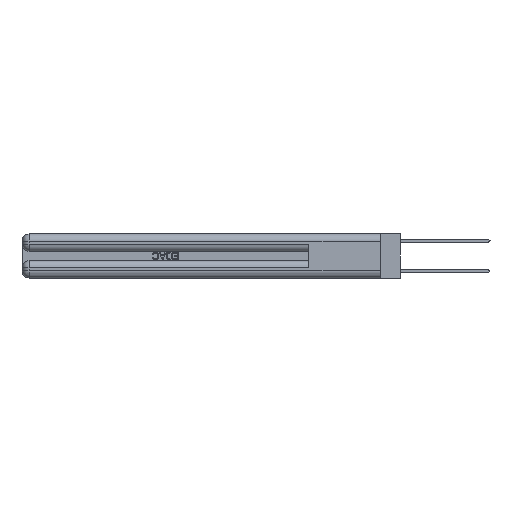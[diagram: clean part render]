
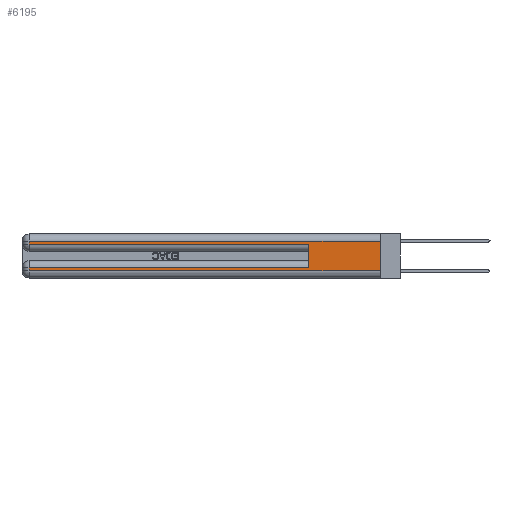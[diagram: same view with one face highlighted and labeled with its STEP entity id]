
A CAD part, left-side view. The second image highlights one B-rep face of the part: STEP entity #6195.
In plain terms, the highlighted planar face has unit normal (-1, 0, 0).
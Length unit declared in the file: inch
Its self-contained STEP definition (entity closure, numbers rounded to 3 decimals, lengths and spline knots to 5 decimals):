
#131 = VECTOR ( 'NONE', #19926, 39.37008 ) ;
#1336 = VECTOR ( 'NONE', #4763, 39.37008 ) ;
#2114 = FACE_OUTER_BOUND ( 'NONE', #22608, .T. ) ;
#2852 = ORIENTED_EDGE ( 'NONE', *, *, #32430, .T. ) ;
#2942 = CARTESIAN_POINT ( 'NONE',  ( 0., 0.6, 0.145 ) ) ;
#3414 = EDGE_CURVE ( 'NONE', #29558, #13386, #12437, .T. ) ;
#4321 = ORIENTED_EDGE ( 'NONE', *, *, #25272, .T. ) ;
#4763 = DIRECTION ( 'NONE',  ( 0., -1., 0. ) ) ;
#5176 = CARTESIAN_POINT ( 'NONE',  ( 0., 0.6, 0.085 ) ) ;
#6195 = ADVANCED_FACE ( 'NONE', ( #2114 ), #9918, .F. ) ;
#6323 = EDGE_CURVE ( 'NONE', #16266, #29972, #7254, .T. ) ;
#7254 = LINE ( 'NONE', #17371, #1336 ) ;
#7320 = ORIENTED_EDGE ( 'NONE', *, *, #3414, .T. ) ;
#8035 = ORIENTED_EDGE ( 'NONE', *, *, #6323, .T. ) ;
#8230 = DIRECTION ( 'NONE',  ( 0., 0., 1. ) ) ;
#8285 = CARTESIAN_POINT ( 'NONE',  ( 0., 2.94, 0.37 ) ) ;
#8598 = DIRECTION ( 'NONE',  ( 0., -1., 0. ) ) ;
#8967 = VERTEX_POINT ( 'NONE', #19197 ) ;
#9192 = EDGE_CURVE ( 'NONE', #29558, #8967, #27785, .T. ) ;
#9569 = VECTOR ( 'NONE', #25282, 39.37008 ) ;
#9840 = LINE ( 'NONE', #12321, #131 ) ;
#9918 = PLANE ( 'NONE',  #19857 ) ;
#9964 = CARTESIAN_POINT ( 'NONE',  ( 0., 0., 0.085 ) ) ;
#10027 = CARTESIAN_POINT ( 'NONE',  ( 0., 2.94, 0.085 ) ) ;
#10107 = VECTOR ( 'NONE', #22360, 39.37008 ) ;
#10209 = VERTEX_POINT ( 'NONE', #16473 ) ;
#10332 = DIRECTION ( 'NONE',  ( 0., 0., -1. ) ) ;
#10405 = LINE ( 'NONE', #15063, #14981 ) ;
#10663 = VECTOR ( 'NONE', #25517, 39.37008 ) ;
#10848 = CARTESIAN_POINT ( 'NONE',  ( 0., 2.94, 0.285 ) ) ;
#12321 = CARTESIAN_POINT ( 'NONE',  ( 0., 2.94, 0.37 ) ) ;
#12437 = LINE ( 'NONE', #9964, #10107 ) ;
#12543 = LINE ( 'NONE', #30387, #9569 ) ;
#13386 = VERTEX_POINT ( 'NONE', #10027 ) ;
#14399 = ORIENTED_EDGE ( 'NONE', *, *, #9192, .F. ) ;
#14981 = VECTOR ( 'NONE', #10332, 39.37008 ) ;
#15063 = CARTESIAN_POINT ( 'NONE',  ( 0., 0., 0.37 ) ) ;
#16266 = VERTEX_POINT ( 'NONE', #28032 ) ;
#16473 = CARTESIAN_POINT ( 'NONE',  ( 0., 2.94, 0.31 ) ) ;
#17123 = VERTEX_POINT ( 'NONE', #18314 ) ;
#17371 = CARTESIAN_POINT ( 'NONE',  ( 0., 0., 0.06 ) ) ;
#17834 = VECTOR ( 'NONE', #8598, 39.37008 ) ;
#18314 = CARTESIAN_POINT ( 'NONE',  ( 0., 0., 0.31 ) ) ;
#19032 = LINE ( 'NONE', #28629, #17834 ) ;
#19197 = CARTESIAN_POINT ( 'NONE',  ( 0., 0.6, 0.285 ) ) ;
#19857 = AXIS2_PLACEMENT_3D ( 'NONE', #24818, #22485, #25458 ) ;
#19926 = DIRECTION ( 'NONE',  ( 0., 0., -1. ) ) ;
#21471 = VECTOR ( 'NONE', #8230, 39.37008 ) ;
#21718 = CARTESIAN_POINT ( 'NONE',  ( 0., 0., 0.06 ) ) ;
#22360 = DIRECTION ( 'NONE',  ( 0., 1., 0. ) ) ;
#22485 = DIRECTION ( 'NONE',  ( 1., 0., 0. ) ) ;
#22608 = EDGE_LOOP ( 'NONE', ( #29975, #22685, #26013, #4321, #14399, #7320, #2852, #8035 ) ) ;
#22685 = ORIENTED_EDGE ( 'NONE', *, *, #31322, .T. ) ;
#23199 = EDGE_CURVE ( 'NONE', #10209, #29274, #9840, .T. ) ;
#23626 = EDGE_CURVE ( 'NONE', #17123, #29972, #10405, .T. ) ;
#24818 = CARTESIAN_POINT ( 'NONE',  ( 0., 0., 0.37 ) ) ;
#25272 = EDGE_CURVE ( 'NONE', #29274, #8967, #19032, .T. ) ;
#25282 = DIRECTION ( 'NONE',  ( 0., 1., 0. ) ) ;
#25458 = DIRECTION ( 'NONE',  ( 0., 0., -1. ) ) ;
#25517 = DIRECTION ( 'NONE',  ( 0., 0., -1. ) ) ;
#26013 = ORIENTED_EDGE ( 'NONE', *, *, #23199, .T. ) ;
#27785 = LINE ( 'NONE', #2942, #21471 ) ;
#28032 = CARTESIAN_POINT ( 'NONE',  ( 0., 2.94, 0.06 ) ) ;
#28151 = LINE ( 'NONE', #8285, #10663 ) ;
#28629 = CARTESIAN_POINT ( 'NONE',  ( 0., 0., 0.285 ) ) ;
#29274 = VERTEX_POINT ( 'NONE', #10848 ) ;
#29558 = VERTEX_POINT ( 'NONE', #5176 ) ;
#29972 = VERTEX_POINT ( 'NONE', #21718 ) ;
#29975 = ORIENTED_EDGE ( 'NONE', *, *, #23626, .F. ) ;
#30387 = CARTESIAN_POINT ( 'NONE',  ( 0., 0., 0.31 ) ) ;
#31322 = EDGE_CURVE ( 'NONE', #17123, #10209, #12543, .T. ) ;
#32430 = EDGE_CURVE ( 'NONE', #13386, #16266, #28151, .T. ) ;
